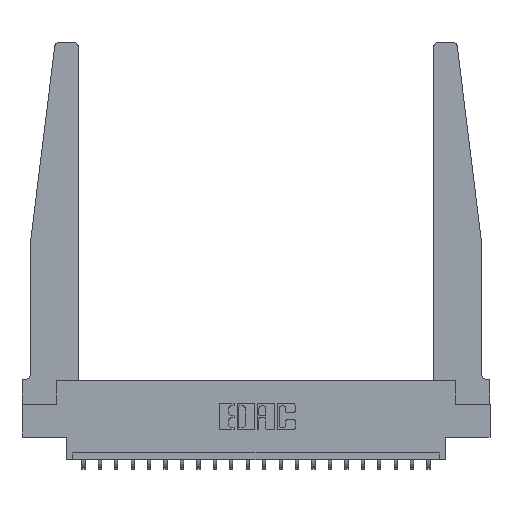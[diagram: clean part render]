
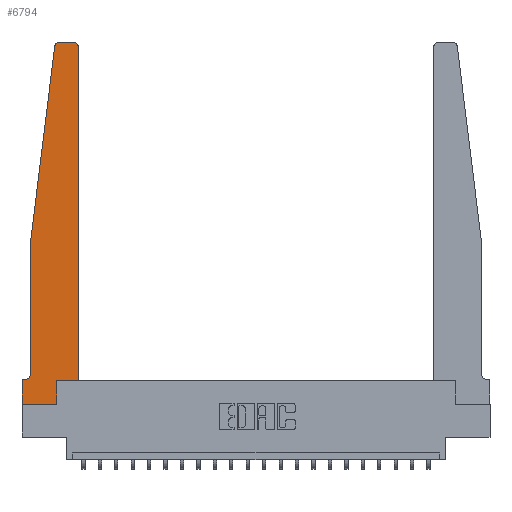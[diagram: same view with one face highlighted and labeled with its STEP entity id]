
A CAD part, top view. The second image highlights one B-rep face of the part: STEP entity #6794.
In plain terms, the highlighted planar face has unit normal (0, 0, 1).
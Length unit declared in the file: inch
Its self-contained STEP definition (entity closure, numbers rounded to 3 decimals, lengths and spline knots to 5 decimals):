
#397 = CARTESIAN_POINT ( 'NONE',  ( 0.24675, 2.72367, 0.37 ) ) ;
#576 = VECTOR ( 'NONE', #7538, 39.37008 ) ;
#608 = CARTESIAN_POINT ( 'NONE',  ( 0.425, 0.18, 0.37 ) ) ;
#662 = VERTEX_POINT ( 'NONE', #10737 ) ;
#848 = ORIENTED_EDGE ( 'NONE', *, *, #8799, .T. ) ;
#925 = AXIS2_PLACEMENT_3D ( 'NONE', #6085, #17629, #7754 ) ;
#1056 = EDGE_CURVE ( 'NONE', #8358, #15262, #14278, .T. ) ;
#1157 = CARTESIAN_POINT ( 'NONE',  ( 0.015, 0.1875, 0.37 ) ) ;
#1518 = LINE ( 'NONE', #18699, #9814 ) ;
#1577 = VECTOR ( 'NONE', #16703, 39.37008 ) ;
#2316 = CARTESIAN_POINT ( 'NONE',  ( 0.065, 1.25, 0.37 ) ) ;
#2615 = CARTESIAN_POINT ( 'NONE',  ( 0.25, 2.75, 0.37 ) ) ;
#2850 = CARTESIAN_POINT ( 'NONE',  ( 0., 0., 0.37 ) ) ;
#2853 = CIRCLE ( 'NONE', #925, 0.05 ) ;
#3215 = PLANE ( 'NONE',  #9238 ) ;
#3371 = EDGE_CURVE ( 'NONE', #13908, #6953, #16500, .T. ) ;
#3722 = CARTESIAN_POINT ( 'NONE',  ( 0.27653, 2.75, 0.37 ) ) ;
#3785 = EDGE_CURVE ( 'NONE', #14945, #662, #1518, .T. ) ;
#3851 = CARTESIAN_POINT ( 'NONE',  ( 0.065, 0.2375, 0.37 ) ) ;
#3875 = LINE ( 'NONE', #19565, #20383 ) ;
#4110 = CARTESIAN_POINT ( 'NONE',  ( 0.425, 2.72, 0.37 ) ) ;
#4701 = ORIENTED_EDGE ( 'NONE', *, *, #9228, .T. ) ;
#4736 = CARTESIAN_POINT ( 'NONE',  ( 0.425, 0.18, 0.37 ) ) ;
#5129 = CARTESIAN_POINT ( 'NONE',  ( 0.2605, 0.18, 0.37 ) ) ;
#5164 = EDGE_CURVE ( 'NONE', #662, #7921, #5811, .T. ) ;
#5329 = CARTESIAN_POINT ( 'NONE',  ( 0.2605, 0.18, 0.37 ) ) ;
#5445 = ORIENTED_EDGE ( 'NONE', *, *, #13076, .T. ) ;
#5477 = FACE_OUTER_BOUND ( 'NONE', #16813, .T. ) ;
#5703 = VECTOR ( 'NONE', #19571, 39.37008 ) ;
#5811 = LINE ( 'NONE', #2850, #19481 ) ;
#5942 = LINE ( 'NONE', #5129, #1577 ) ;
#6085 = CARTESIAN_POINT ( 'NONE',  ( 0.015, 0.2375, 0.37 ) ) ;
#6178 = ORIENTED_EDGE ( 'NONE', *, *, #3785, .T. ) ;
#6322 = ORIENTED_EDGE ( 'NONE', *, *, #5164, .T. ) ;
#6794 = ADVANCED_FACE ( 'NONE', ( #5477 ), #3215, .T. ) ;
#6953 = VERTEX_POINT ( 'NONE', #608 ) ;
#7074 = ORIENTED_EDGE ( 'NONE', *, *, #20942, .T. ) ;
#7401 = DIRECTION ( 'NONE',  ( -1., 0., 0. ) ) ;
#7468 = VERTEX_POINT ( 'NONE', #11855 ) ;
#7523 = ORIENTED_EDGE ( 'NONE', *, *, #13346, .T. ) ;
#7538 = DIRECTION ( 'NONE',  ( -1., 0., 0. ) ) ;
#7718 = CARTESIAN_POINT ( 'NONE',  ( 0.425, 0.18, 0.37 ) ) ;
#7754 = DIRECTION ( 'NONE',  ( -1., 0., 0. ) ) ;
#7921 = VERTEX_POINT ( 'NONE', #8011 ) ;
#7997 = DIRECTION ( 'NONE',  ( 1., 0., 0. ) ) ;
#8011 = CARTESIAN_POINT ( 'NONE',  ( 0., 0., 0.37 ) ) ;
#8205 = DIRECTION ( 'NONE',  ( 0., 0., 1. ) ) ;
#8358 = VERTEX_POINT ( 'NONE', #18916 ) ;
#8500 = VECTOR ( 'NONE', #9068, 39.37008 ) ;
#8799 = EDGE_CURVE ( 'NONE', #7468, #15341, #9552, .T. ) ;
#8813 = CARTESIAN_POINT ( 'NONE',  ( 0.395, 2.72, 0.37 ) ) ;
#9068 = DIRECTION ( 'NONE',  ( 0., -1., 0. ) ) ;
#9182 = AXIS2_PLACEMENT_3D ( 'NONE', #8813, #20308, #10495 ) ;
#9228 = EDGE_CURVE ( 'NONE', #11584, #7468, #10062, .T. ) ;
#9238 = AXIS2_PLACEMENT_3D ( 'NONE', #21314, #8205, #19700 ) ;
#9406 = CARTESIAN_POINT ( 'NONE',  ( 0.27653, 2.72, 0.37 ) ) ;
#9552 = LINE ( 'NONE', #13961, #8500 ) ;
#9790 = EDGE_CURVE ( 'NONE', #13619, #8358, #17200, .T. ) ;
#9814 = VECTOR ( 'NONE', #7401, 39.37008 ) ;
#10062 = LINE ( 'NONE', #2316, #14931 ) ;
#10159 = LINE ( 'NONE', #4736, #5703 ) ;
#10495 = DIRECTION ( 'NONE',  ( 1., 0., 0. ) ) ;
#10737 = CARTESIAN_POINT ( 'NONE',  ( 0., 0.1875, 0.37 ) ) ;
#11055 = DIRECTION ( 'NONE',  ( 1., 0., 0. ) ) ;
#11584 = VERTEX_POINT ( 'NONE', #397 ) ;
#11855 = CARTESIAN_POINT ( 'NONE',  ( 0.065, 1.25, 0.37 ) ) ;
#11945 = ORIENTED_EDGE ( 'NONE', *, *, #1056, .T. ) ;
#12097 = VECTOR ( 'NONE', #12705, 39.37008 ) ;
#12216 = DIRECTION ( 'NONE',  ( -0.122, -0.992, 0. ) ) ;
#12653 = EDGE_CURVE ( 'NONE', #6953, #13619, #10159, .T. ) ;
#12705 = DIRECTION ( 'NONE',  ( 1., 0., 0. ) ) ;
#13076 = EDGE_CURVE ( 'NONE', #15341, #14945, #2853, .T. ) ;
#13346 = EDGE_CURVE ( 'NONE', #16604, #13908, #5942, .T. ) ;
#13413 = CIRCLE ( 'NONE', #18463, 0.03 ) ;
#13577 = CARTESIAN_POINT ( 'NONE',  ( 0.2605, 0., 0.37 ) ) ;
#13619 = VERTEX_POINT ( 'NONE', #4110 ) ;
#13908 = VERTEX_POINT ( 'NONE', #5329 ) ;
#13961 = CARTESIAN_POINT ( 'NONE',  ( 0.065, 1.25, 0.37 ) ) ;
#14078 = ORIENTED_EDGE ( 'NONE', *, *, #3371, .T. ) ;
#14180 = EDGE_CURVE ( 'NONE', #15262, #11584, #13413, .T. ) ;
#14278 = LINE ( 'NONE', #2615, #576 ) ;
#14433 = DIRECTION ( 'NONE',  ( 0., -1., 0. ) ) ;
#14931 = VECTOR ( 'NONE', #12216, 39.37008 ) ;
#14945 = VERTEX_POINT ( 'NONE', #1157 ) ;
#15262 = VERTEX_POINT ( 'NONE', #3722 ) ;
#15341 = VERTEX_POINT ( 'NONE', #3851 ) ;
#16500 = LINE ( 'NONE', #7718, #12097 ) ;
#16604 = VERTEX_POINT ( 'NONE', #13577 ) ;
#16703 = DIRECTION ( 'NONE',  ( 0., 1., 0. ) ) ;
#16813 = EDGE_LOOP ( 'NONE', ( #11945, #16850, #4701, #848, #5445, #6178, #6322, #7074, #7523, #14078, #17210, #17053 ) ) ;
#16850 = ORIENTED_EDGE ( 'NONE', *, *, #14180, .T. ) ;
#17053 = ORIENTED_EDGE ( 'NONE', *, *, #9790, .T. ) ;
#17200 = CIRCLE ( 'NONE', #9182, 0.03 ) ;
#17210 = ORIENTED_EDGE ( 'NONE', *, *, #12653, .T. ) ;
#17629 = DIRECTION ( 'NONE',  ( 0., 0., -1. ) ) ;
#18463 = AXIS2_PLACEMENT_3D ( 'NONE', #9406, #20895, #11055 ) ;
#18699 = CARTESIAN_POINT ( 'NONE',  ( 0.065, 0.1875, 0.37 ) ) ;
#18916 = CARTESIAN_POINT ( 'NONE',  ( 0.395, 2.75, 0.37 ) ) ;
#19481 = VECTOR ( 'NONE', #14433, 39.37008 ) ;
#19565 = CARTESIAN_POINT ( 'NONE',  ( 0., 0., 0.37 ) ) ;
#19571 = DIRECTION ( 'NONE',  ( 0., 1., 0. ) ) ;
#19700 = DIRECTION ( 'NONE',  ( 1., 0., 0. ) ) ;
#20308 = DIRECTION ( 'NONE',  ( 0., 0., 1. ) ) ;
#20383 = VECTOR ( 'NONE', #7997, 39.37008 ) ;
#20895 = DIRECTION ( 'NONE',  ( 0., 0., 1. ) ) ;
#20942 = EDGE_CURVE ( 'NONE', #7921, #16604, #3875, .T. ) ;
#21314 = CARTESIAN_POINT ( 'NONE',  ( 0., 0.1875, 0.37 ) ) ;
